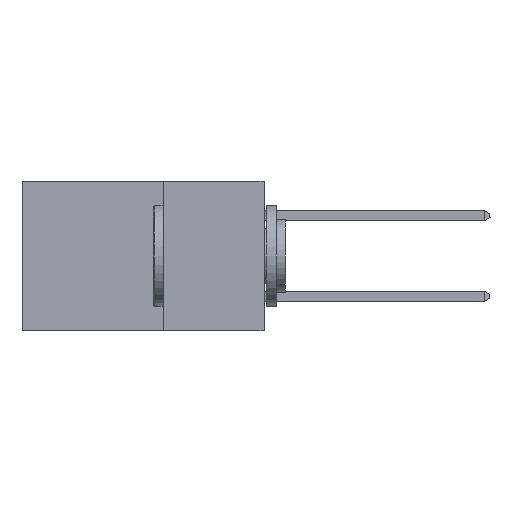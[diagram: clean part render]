
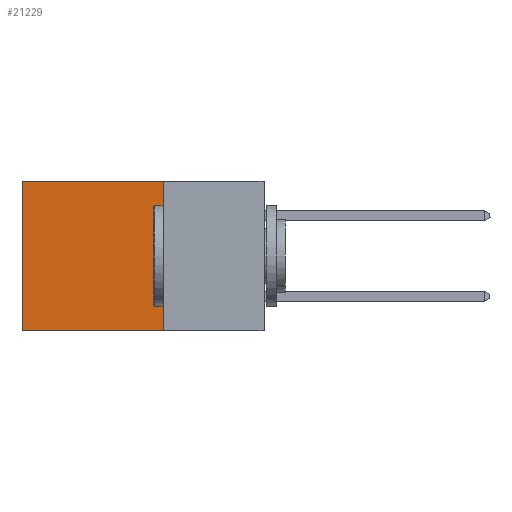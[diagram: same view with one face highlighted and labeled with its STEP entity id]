
A CAD part, left-side view. The second image highlights one B-rep face of the part: STEP entity #21229.
In plain terms, the highlighted planar face has unit normal (-1, 0, 0).
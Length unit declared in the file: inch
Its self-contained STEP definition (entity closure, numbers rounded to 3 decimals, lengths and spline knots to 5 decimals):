
#89 = VERTEX_POINT ( 'NONE', #20181 ) ;
#447 = CARTESIAN_POINT ( 'NONE',  ( 0.298, 0.6, 0. ) ) ;
#586 = ORIENTED_EDGE ( 'NONE', *, *, #15504, .T. ) ;
#669 = DIRECTION ( 'NONE',  ( 1., 0., 0. ) ) ;
#1255 = ORIENTED_EDGE ( 'NONE', *, *, #18320, .F. ) ;
#1931 = LINE ( 'NONE', #17443, #2479 ) ;
#2479 = VECTOR ( 'NONE', #12088, 39.37008 ) ;
#4149 = EDGE_LOOP ( 'NONE', ( #586, #1255, #8824, #9642 ) ) ;
#4351 = EDGE_CURVE ( 'NONE', #20995, #89, #16925, .T. ) ;
#4778 = CARTESIAN_POINT ( 'NONE',  ( 0.298, 0.25, -0.37 ) ) ;
#6316 = DIRECTION ( 'NONE',  ( 0., 0., -1. ) ) ;
#7648 = AXIS2_PLACEMENT_3D ( 'NONE', #11605, #669, #13376 ) ;
#8118 = VERTEX_POINT ( 'NONE', #447 ) ;
#8324 = CARTESIAN_POINT ( 'NONE',  ( 0.298, 0.25, 0. ) ) ;
#8744 = CARTESIAN_POINT ( 'NONE',  ( 0.298, 0.25, 0. ) ) ;
#8824 = ORIENTED_EDGE ( 'NONE', *, *, #4351, .F. ) ;
#9642 = ORIENTED_EDGE ( 'NONE', *, *, #18036, .T. ) ;
#11605 = CARTESIAN_POINT ( 'NONE',  ( 0.298, 0.25, 0. ) ) ;
#12038 = FACE_OUTER_BOUND ( 'NONE', #4149, .T. ) ;
#12088 = DIRECTION ( 'NONE',  ( 0., 0., -1. ) ) ;
#13376 = DIRECTION ( 'NONE',  ( 0., 0., -1. ) ) ;
#13495 = VERTEX_POINT ( 'NONE', #17460 ) ;
#14947 = VECTOR ( 'NONE', #17480, 39.37008 ) ;
#15504 = EDGE_CURVE ( 'NONE', #8118, #13495, #1931, .T. ) ;
#16675 = LINE ( 'NONE', #4778, #14947 ) ;
#16925 = LINE ( 'NONE', #8324, #17813 ) ;
#17191 = PLANE ( 'NONE',  #7648 ) ;
#17443 = CARTESIAN_POINT ( 'NONE',  ( 0.298, 0.6, 0. ) ) ;
#17460 = CARTESIAN_POINT ( 'NONE',  ( 0.298, 0.6, -0.37 ) ) ;
#17480 = DIRECTION ( 'NONE',  ( 0., 1., 0. ) ) ;
#17555 = VECTOR ( 'NONE', #19699, 39.37008 ) ;
#17813 = VECTOR ( 'NONE', #6316, 39.37008 ) ;
#18036 = EDGE_CURVE ( 'NONE', #20995, #8118, #18721, .T. ) ;
#18320 = EDGE_CURVE ( 'NONE', #89, #13495, #16675, .T. ) ;
#18721 = LINE ( 'NONE', #8744, #17555 ) ;
#19699 = DIRECTION ( 'NONE',  ( 0., 1., 0. ) ) ;
#20181 = CARTESIAN_POINT ( 'NONE',  ( 0.298, 0.25, -0.37 ) ) ;
#20505 = CARTESIAN_POINT ( 'NONE',  ( 0.298, 0.25, 0. ) ) ;
#20995 = VERTEX_POINT ( 'NONE', #20505 ) ;
#21229 = ADVANCED_FACE ( 'NONE', ( #12038 ), #17191, .F. ) ;
